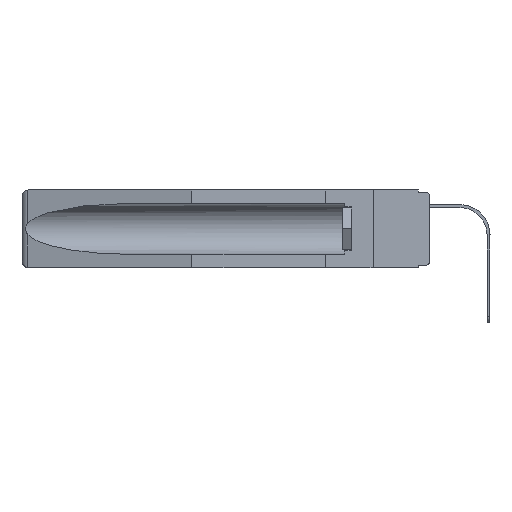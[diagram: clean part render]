
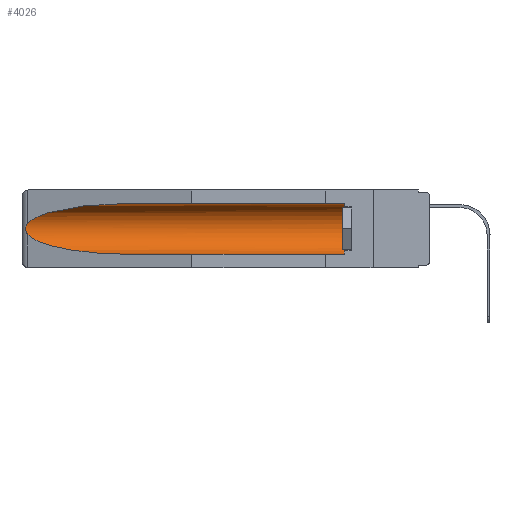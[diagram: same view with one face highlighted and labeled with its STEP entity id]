
A CAD part, left-side view. The second image highlights one B-rep face of the part: STEP entity #4026.
In plain terms, the highlighted cylindrical face has radius 2.857 mm (diameter 5.715 mm), a partial arc.
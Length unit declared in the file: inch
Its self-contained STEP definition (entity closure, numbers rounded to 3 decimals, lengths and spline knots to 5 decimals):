
#240 = CARTESIAN_POINT ( 'NONE',  ( 0.155, 1.07973, -0.284 ) ) ;
#885 = CARTESIAN_POINT ( 'NONE',  ( 0.21114, 1.30732, -0.059 ) ) ;
#976 = DIRECTION ( 'NONE',  ( 0., 0., 1. ) ) ;
#1079 = EDGE_LOOP ( 'NONE', ( #14302, #10652, #16080, #6352, #8219, #4652 ) ) ;
#1850 = CARTESIAN_POINT ( 'NONE',  ( 0.26537, 1.52718, -0.19328 ) ) ;
#2429 = CARTESIAN_POINT ( 'NONE',  ( 0.26597, 1.5296, -0.19026 ) ) ;
#2590 = DIRECTION ( 'NONE',  ( 0., 1., 0. ) ) ;
#2878 = DIRECTION ( 'NONE',  ( 0., 0., 1. ) ) ;
#3359 =( BOUNDED_CURVE ( )  B_SPLINE_CURVE ( 3, ( #3968, #885, #6937, #7125 ),
 .UNSPECIFIED., .F., .T. ) 
 B_SPLINE_CURVE_WITH_KNOTS ( ( 4, 4 ),
 ( 4.71239, 6.08839 ),
 .UNSPECIFIED. ) 
 CURVE ( )  GEOMETRIC_REPRESENTATION_ITEM ( )  RATIONAL_B_SPLINE_CURVE ( ( 1., 0.848, 0.848, 1. ) ) 
 REPRESENTATION_ITEM ( '' )  );
#3841 = CARTESIAN_POINT ( 'NONE',  ( 0.155, -0.30754, -0.059 ) ) ;
#3968 = CARTESIAN_POINT ( 'NONE',  ( 0.155, 1.07973, -0.059 ) ) ;
#4026 = ADVANCED_FACE ( 'NONE', ( #10272 ), #13817, .F. ) ;
#4327 = DIRECTION ( 'NONE',  ( 0., 1., 0. ) ) ;
#4467 = VERTEX_POINT ( 'NONE', #16227 ) ;
#4650 = VECTOR ( 'NONE', #4327, 39.37008 ) ;
#4652 = ORIENTED_EDGE ( 'NONE', *, *, #17064, .T. ) ;
#4742 = CARTESIAN_POINT ( 'NONE',  ( 0.155, 1.07973, -0.284 ) ) ;
#5223 = CARTESIAN_POINT ( 'NONE',  ( 0.2673, 1.5327, -0.16383 ) ) ;
#5235 = VERTEX_POINT ( 'NONE', #12814 ) ;
#5520 = CARTESIAN_POINT ( 'NONE',  ( 0.26655, 1.53094, -0.18657 ) ) ;
#5856 = VERTEX_POINT ( 'NONE', #11307 ) ;
#6255 = CARTESIAN_POINT ( 'NONE',  ( 0.155, 0.126, -0.284 ) ) ;
#6352 = ORIENTED_EDGE ( 'NONE', *, *, #11271, .F. ) ;
#6686 = EDGE_CURVE ( 'NONE', #4467, #8210, #18748, .T. ) ;
#6937 = CARTESIAN_POINT ( 'NONE',  ( 0.25451, 1.48313, -0.09465 ) ) ;
#7065 = EDGE_CURVE ( 'NONE', #5235, #4467, #15744, .T. ) ;
#7125 = CARTESIAN_POINT ( 'NONE',  ( 0.26537, 1.52718, -0.14972 ) ) ;
#8210 = VERTEX_POINT ( 'NONE', #240 ) ;
#8219 = ORIENTED_EDGE ( 'NONE', *, *, #19024, .T. ) ;
#9490 = CIRCLE ( 'NONE', #10469, 0.1125 ) ;
#9764 = CARTESIAN_POINT ( 'NONE',  ( 0.155, 1.07973, -0.059 ) ) ;
#10272 = FACE_OUTER_BOUND ( 'NONE', #1079, .T. ) ;
#10469 = AXIS2_PLACEMENT_3D ( 'NONE', #19934, #20032, #2878 ) ;
#10569 = EDGE_CURVE ( 'NONE', #13466, #5235, #3359, .T. ) ;
#10652 = ORIENTED_EDGE ( 'NONE', *, *, #7065, .T. ) ;
#11271 = EDGE_CURVE ( 'NONE', #16499, #8210, #16474, .T. ) ;
#11307 = CARTESIAN_POINT ( 'NONE',  ( 0.155, 0.126, -0.059 ) ) ;
#11427 = CARTESIAN_POINT ( 'NONE',  ( 0.2675, 1.53308, -0.16763 ) ) ;
#11968 = CARTESIAN_POINT ( 'NONE',  ( 0.155, -0.30754, -0.284 ) ) ;
#12814 = CARTESIAN_POINT ( 'NONE',  ( 0.26537, 1.52718, -0.14972 ) ) ;
#13074 = CARTESIAN_POINT ( 'NONE',  ( 0.2675, 1.53308, -0.17534 ) ) ;
#13172 = CARTESIAN_POINT ( 'NONE',  ( 0.26537, 1.52718, -0.14972 ) ) ;
#13263 = CARTESIAN_POINT ( 'NONE',  ( 0.26597, 1.52961, -0.15275 ) ) ;
#13466 = VERTEX_POINT ( 'NONE', #9764 ) ;
#13660 = VECTOR ( 'NONE', #2590, 39.37008 ) ;
#13817 = CYLINDRICAL_SURFACE ( 'NONE', #14725, 0.1125 ) ;
#14302 = ORIENTED_EDGE ( 'NONE', *, *, #10569, .T. ) ;
#14725 = AXIS2_PLACEMENT_3D ( 'NONE', #20044, #18610, #976 ) ;
#15744 = B_SPLINE_CURVE_WITH_KNOTS ( 'NONE', 3,
 ( #13172, #13263, #19392, #5223, #11427, #13074, #19589, #5520, #2429, #19290 ),
 .UNSPECIFIED., .F., .F.,
 ( 4, 2, 2, 2, 4 ),
 ( 0., 0.00029, 0.00058, 0.00087, 0.00117 ),
 .UNSPECIFIED. ) ;
#16080 = ORIENTED_EDGE ( 'NONE', *, *, #6686, .T. ) ;
#16227 = CARTESIAN_POINT ( 'NONE',  ( 0.26537, 1.52718, -0.19328 ) ) ;
#16474 = LINE ( 'NONE', #11968, #4650 ) ;
#16499 = VERTEX_POINT ( 'NONE', #6255 ) ;
#17064 = EDGE_CURVE ( 'NONE', #5856, #13466, #19450, .T. ) ;
#17088 = CARTESIAN_POINT ( 'NONE',  ( 0.21114, 1.30732, -0.284 ) ) ;
#18610 = DIRECTION ( 'NONE',  ( 0., 1., 0. ) ) ;
#18748 =( BOUNDED_CURVE ( )  B_SPLINE_CURVE ( 3, ( #1850, #19022, #17088, #4742 ),
 .UNSPECIFIED., .F., .T. ) 
 B_SPLINE_CURVE_WITH_KNOTS ( ( 4, 4 ),
 ( 0.1948, 1.5708 ),
 .UNSPECIFIED. ) 
 CURVE ( )  GEOMETRIC_REPRESENTATION_ITEM ( )  RATIONAL_B_SPLINE_CURVE ( ( 1., 0.848, 0.848, 1. ) ) 
 REPRESENTATION_ITEM ( '' )  );
#19022 = CARTESIAN_POINT ( 'NONE',  ( 0.25451, 1.48313, -0.24835 ) ) ;
#19024 = EDGE_CURVE ( 'NONE', #16499, #5856, #9490, .T. ) ;
#19290 = CARTESIAN_POINT ( 'NONE',  ( 0.26537, 1.52718, -0.19328 ) ) ;
#19392 = CARTESIAN_POINT ( 'NONE',  ( 0.26654, 1.53092, -0.15636 ) ) ;
#19450 = LINE ( 'NONE', #3841, #13660 ) ;
#19589 = CARTESIAN_POINT ( 'NONE',  ( 0.2673, 1.53269, -0.17917 ) ) ;
#19934 = CARTESIAN_POINT ( 'NONE',  ( 0.155, 0.126, -0.1715 ) ) ;
#20032 = DIRECTION ( 'NONE',  ( 0., -1., 0. ) ) ;
#20044 = CARTESIAN_POINT ( 'NONE',  ( 0.155, -0.30754, -0.1715 ) ) ;
